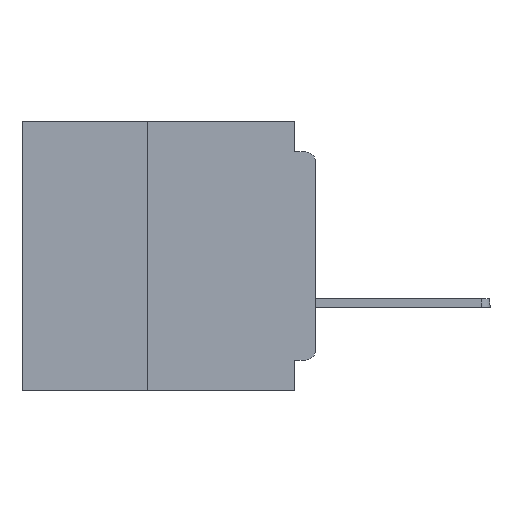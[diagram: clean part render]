
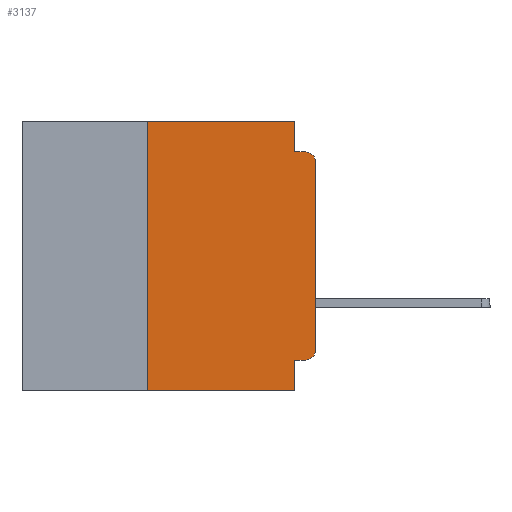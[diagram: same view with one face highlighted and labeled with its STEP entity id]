
A CAD part, left-side view. The second image highlights one B-rep face of the part: STEP entity #3137.
In plain terms, the highlighted planar face has unit normal (-1, 0, 0).
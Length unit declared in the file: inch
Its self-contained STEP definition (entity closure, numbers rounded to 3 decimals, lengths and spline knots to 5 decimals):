
#143 = DIRECTION ( 'NONE',  ( 0., 0., -1. ) ) ;
#513 = CARTESIAN_POINT ( 'NONE',  ( 0., 0.031, -0.045 ) ) ;
#681 = EDGE_CURVE ( 'NONE', #17076, #14165, #18018, .T. ) ;
#2576 = LINE ( 'NONE', #22857, #10122 ) ;
#3137 = ADVANCED_FACE ( 'NONE', ( #21650 ), #34898, .F. ) ;
#4297 = EDGE_CURVE ( 'NONE', #16877, #26541, #2576, .T. ) ;
#4470 = EDGE_CURVE ( 'NONE', #20348, #33800, #9657, .T. ) ;
#4934 = DIRECTION ( 'NONE',  ( 0., 0., -1. ) ) ;
#5836 = EDGE_CURVE ( 'NONE', #9393, #33800, #8656, .T. ) ;
#6835 = CARTESIAN_POINT ( 'NONE',  ( 0., 0.031, -0.4 ) ) ;
#7565 = LINE ( 'NONE', #13571, #21666 ) ;
#8199 = CIRCLE ( 'NONE', #20143, 0.015 ) ;
#8656 = LINE ( 'NONE', #16403, #15310 ) ;
#8955 = ORIENTED_EDGE ( 'NONE', *, *, #28749, .F. ) ;
#9393 = VERTEX_POINT ( 'NONE', #18131 ) ;
#9443 = VECTOR ( 'NONE', #21083, 39.37008 ) ;
#9657 = LINE ( 'NONE', #19554, #18085 ) ;
#9813 = ORIENTED_EDGE ( 'NONE', *, *, #5836, .T. ) ;
#10122 = VECTOR ( 'NONE', #22965, 39.37008 ) ;
#11235 = ORIENTED_EDGE ( 'NONE', *, *, #17894, .F. ) ;
#11520 = LINE ( 'NONE', #26244, #32843 ) ;
#11921 = EDGE_CURVE ( 'NONE', #14165, #26874, #31675, .T. ) ;
#12006 = CARTESIAN_POINT ( 'NONE',  ( 0., 0., -0.34 ) ) ;
#12718 = DIRECTION ( 'NONE',  ( -1., 0., 0. ) ) ;
#13146 = ORIENTED_EDGE ( 'NONE', *, *, #4297, .T. ) ;
#13571 = CARTESIAN_POINT ( 'NONE',  ( 0., 0.25, -0.4 ) ) ;
#13801 = CARTESIAN_POINT ( 'NONE',  ( 0., 0.015, -0.045 ) ) ;
#13909 = VECTOR ( 'NONE', #19858, 39.37008 ) ;
#14165 = VERTEX_POINT ( 'NONE', #513 ) ;
#15310 = VECTOR ( 'NONE', #16567, 39.37008 ) ;
#15502 = EDGE_CURVE ( 'NONE', #16552, #16877, #8199, .T. ) ;
#15571 = CIRCLE ( 'NONE', #32478, 0.015 ) ;
#15705 = CARTESIAN_POINT ( 'NONE',  ( 0., 0.031, 0. ) ) ;
#16154 = AXIS2_PLACEMENT_3D ( 'NONE', #33602, #33562, #33467 ) ;
#16240 = VECTOR ( 'NONE', #4934, 39.37008 ) ;
#16403 = CARTESIAN_POINT ( 'NONE',  ( 0., 0.437, -0.4 ) ) ;
#16454 = DIRECTION ( 'NONE',  ( 0., 0., 1. ) ) ;
#16552 = VERTEX_POINT ( 'NONE', #30067 ) ;
#16567 = DIRECTION ( 'NONE',  ( 0., -1., 0. ) ) ;
#16877 = VERTEX_POINT ( 'NONE', #12006 ) ;
#17064 = DIRECTION ( 'NONE',  ( -1., 0., 0. ) ) ;
#17076 = VERTEX_POINT ( 'NONE', #15705 ) ;
#17095 = CARTESIAN_POINT ( 'NONE',  ( 0., 0., -0.355 ) ) ;
#17714 = EDGE_CURVE ( 'NONE', #26541, #26874, #15571, .T. ) ;
#17894 = EDGE_CURVE ( 'NONE', #9393, #33772, #7565, .T. ) ;
#18018 = LINE ( 'NONE', #20942, #16240 ) ;
#18085 = VECTOR ( 'NONE', #19616, 39.37008 ) ;
#18131 = CARTESIAN_POINT ( 'NONE',  ( 0., 0.25, -0.4 ) ) ;
#18309 = CARTESIAN_POINT ( 'NONE',  ( 0., 0., -0.045 ) ) ;
#19554 = CARTESIAN_POINT ( 'NONE',  ( 0., 0.031, -0.4 ) ) ;
#19616 = DIRECTION ( 'NONE',  ( 0., 0., -1. ) ) ;
#19858 = DIRECTION ( 'NONE',  ( 0., 1., 0. ) ) ;
#20143 = AXIS2_PLACEMENT_3D ( 'NONE', #33629, #17064, #143 ) ;
#20348 = VERTEX_POINT ( 'NONE', #33510 ) ;
#20942 = CARTESIAN_POINT ( 'NONE',  ( 0., 0.031, 0. ) ) ;
#21083 = DIRECTION ( 'NONE',  ( 0., -1., 0. ) ) ;
#21258 = ORIENTED_EDGE ( 'NONE', *, *, #11921, .F. ) ;
#21650 = FACE_OUTER_BOUND ( 'NONE', #22761, .T. ) ;
#21666 = VECTOR ( 'NONE', #16454, 39.37008 ) ;
#22761 = EDGE_LOOP ( 'NONE', ( #13146, #33783, #21258, #35517, #8955, #11235, #9813, #28641, #23491, #32511 ) ) ;
#22857 = CARTESIAN_POINT ( 'NONE',  ( 0., 0., 0. ) ) ;
#22965 = DIRECTION ( 'NONE',  ( 0., 0., 1. ) ) ;
#23491 = ORIENTED_EDGE ( 'NONE', *, *, #26319, .F. ) ;
#23629 = CARTESIAN_POINT ( 'NONE',  ( 0., 0., -0.06 ) ) ;
#26244 = CARTESIAN_POINT ( 'NONE',  ( 0., 0.437, 0. ) ) ;
#26319 = EDGE_CURVE ( 'NONE', #16552, #20348, #36045, .T. ) ;
#26345 = CARTESIAN_POINT ( 'NONE',  ( 0., 0.25, 0. ) ) ;
#26541 = VERTEX_POINT ( 'NONE', #23629 ) ;
#26874 = VERTEX_POINT ( 'NONE', #13801 ) ;
#28641 = ORIENTED_EDGE ( 'NONE', *, *, #4470, .F. ) ;
#28749 = EDGE_CURVE ( 'NONE', #33772, #17076, #11520, .T. ) ;
#29049 = DIRECTION ( 'NONE',  ( 0., -1., 0. ) ) ;
#29436 = CARTESIAN_POINT ( 'NONE',  ( 0., 0.015, -0.06 ) ) ;
#30067 = CARTESIAN_POINT ( 'NONE',  ( 0., 0.015, -0.355 ) ) ;
#31675 = LINE ( 'NONE', #18309, #9443 ) ;
#32173 = DIRECTION ( 'NONE',  ( 0., 0., -1. ) ) ;
#32478 = AXIS2_PLACEMENT_3D ( 'NONE', #29436, #12718, #32173 ) ;
#32511 = ORIENTED_EDGE ( 'NONE', *, *, #15502, .T. ) ;
#32843 = VECTOR ( 'NONE', #29049, 39.37008 ) ;
#33467 = DIRECTION ( 'NONE',  ( 0., 0., -1. ) ) ;
#33510 = CARTESIAN_POINT ( 'NONE',  ( 0., 0.031, -0.355 ) ) ;
#33562 = DIRECTION ( 'NONE',  ( 1., 0., 0. ) ) ;
#33602 = CARTESIAN_POINT ( 'NONE',  ( 0., 0.437, 0. ) ) ;
#33629 = CARTESIAN_POINT ( 'NONE',  ( 0., 0.015, -0.34 ) ) ;
#33772 = VERTEX_POINT ( 'NONE', #26345 ) ;
#33783 = ORIENTED_EDGE ( 'NONE', *, *, #17714, .T. ) ;
#33800 = VERTEX_POINT ( 'NONE', #6835 ) ;
#34898 = PLANE ( 'NONE',  #16154 ) ;
#35517 = ORIENTED_EDGE ( 'NONE', *, *, #681, .F. ) ;
#36045 = LINE ( 'NONE', #17095, #13909 ) ;
